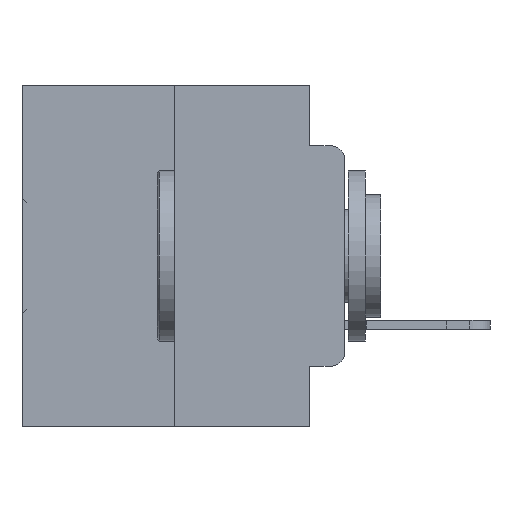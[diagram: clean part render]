
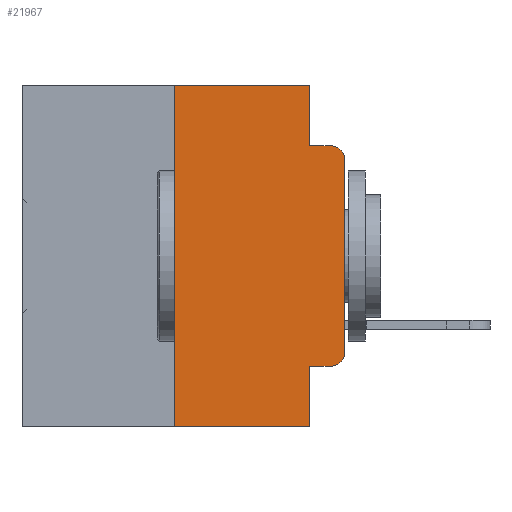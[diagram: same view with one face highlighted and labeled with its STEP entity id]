
A CAD part, left-side view. The second image highlights one B-rep face of the part: STEP entity #21967.
In plain terms, the highlighted planar face has unit normal (-1, 0, 0).
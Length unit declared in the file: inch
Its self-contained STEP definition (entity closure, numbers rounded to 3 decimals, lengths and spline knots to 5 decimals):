
#9 = VECTOR ( 'NONE', #4229, 39.37008 ) ;
#162 = CARTESIAN_POINT ( 'NONE',  ( 0., 0.02, -0.0885 ) ) ;
#544 = CARTESIAN_POINT ( 'NONE',  ( 0., 0.473, -0.5 ) ) ;
#955 = LINE ( 'NONE', #9990, #9 ) ;
#1294 = ORIENTED_EDGE ( 'NONE', *, *, #5233, .T. ) ;
#1301 = EDGE_CURVE ( 'NONE', #25067, #18121, #32354, .T. ) ;
#3292 = ORIENTED_EDGE ( 'NONE', *, *, #1301, .T. ) ;
#3475 = VERTEX_POINT ( 'NONE', #28756 ) ;
#3494 = DIRECTION ( 'NONE',  ( 0., -1., 0. ) ) ;
#4229 = DIRECTION ( 'NONE',  ( 0., -1., 0. ) ) ;
#4301 = VERTEX_POINT ( 'NONE', #18008 ) ;
#4557 = LINE ( 'NONE', #26283, #11226 ) ;
#4990 = ORIENTED_EDGE ( 'NONE', *, *, #32111, .F. ) ;
#5233 = EDGE_CURVE ( 'NONE', #30755, #25067, #18226, .T. ) ;
#5246 = ORIENTED_EDGE ( 'NONE', *, *, #25232, .F. ) ;
#5664 = VERTEX_POINT ( 'NONE', #18319 ) ;
#7250 = CARTESIAN_POINT ( 'NONE',  ( 0., 0.473, 0. ) ) ;
#8389 = EDGE_CURVE ( 'NONE', #4301, #11803, #9039, .T. ) ;
#8598 = LINE ( 'NONE', #19169, #34910 ) ;
#9039 = CIRCLE ( 'NONE', #10577, 0.02 ) ;
#9617 = CARTESIAN_POINT ( 'NONE',  ( 0., 0.02, -0.4115 ) ) ;
#9990 = CARTESIAN_POINT ( 'NONE',  ( 0., 0.473, 0. ) ) ;
#10044 = DIRECTION ( 'NONE',  ( 0., 0., 1. ) ) ;
#10074 = DIRECTION ( 'NONE',  ( 1., 0., 0. ) ) ;
#10155 = VECTOR ( 'NONE', #30613, 39.37008 ) ;
#10577 = AXIS2_PLACEMENT_3D ( 'NONE', #11622, #11499, #11469 ) ;
#10914 = EDGE_CURVE ( 'NONE', #30755, #3475, #26461, .T. ) ;
#11226 = VECTOR ( 'NONE', #28831, 39.37008 ) ;
#11469 = DIRECTION ( 'NONE',  ( 0., 0., -1. ) ) ;
#11499 = DIRECTION ( 'NONE',  ( -1., 0., 0. ) ) ;
#11622 = CARTESIAN_POINT ( 'NONE',  ( 0., 0.02, -0.1085 ) ) ;
#11803 = VERTEX_POINT ( 'NONE', #162 ) ;
#12733 = EDGE_CURVE ( 'NONE', #5664, #14747, #30363, .T. ) ;
#13127 = VECTOR ( 'NONE', #3494, 39.37008 ) ;
#13420 = DIRECTION ( 'NONE',  ( 0., 0., -1. ) ) ;
#13431 = CARTESIAN_POINT ( 'NONE',  ( 0., 0.051, 0. ) ) ;
#13567 = ORIENTED_EDGE ( 'NONE', *, *, #26563, .F. ) ;
#13974 = CARTESIAN_POINT ( 'NONE',  ( 0., 0., -0.3915 ) ) ;
#14747 = VERTEX_POINT ( 'NONE', #23717 ) ;
#15728 = EDGE_CURVE ( 'NONE', #18121, #4301, #8598, .T. ) ;
#16088 = CARTESIAN_POINT ( 'NONE',  ( 0., 0.051, 0. ) ) ;
#18008 = CARTESIAN_POINT ( 'NONE',  ( 0., 0., -0.1085 ) ) ;
#18121 = VERTEX_POINT ( 'NONE', #13974 ) ;
#18226 = LINE ( 'NONE', #30571, #10155 ) ;
#18319 = CARTESIAN_POINT ( 'NONE',  ( 0., 0.25, -0.5 ) ) ;
#19169 = CARTESIAN_POINT ( 'NONE',  ( 0., 0., 0. ) ) ;
#19987 = VERTEX_POINT ( 'NONE', #16088 ) ;
#20302 = VECTOR ( 'NONE', #13420, 39.37008 ) ;
#20640 = CARTESIAN_POINT ( 'NONE',  ( 0., 0.02, -0.3915 ) ) ;
#21967 = ADVANCED_FACE ( 'NONE', ( #34445 ), #23293, .F. ) ;
#22881 = ORIENTED_EDGE ( 'NONE', *, *, #15728, .T. ) ;
#23192 = EDGE_LOOP ( 'NONE', ( #22881, #25909, #4990, #5246, #13567, #23478, #29846, #33278, #1294, #3292 ) ) ;
#23293 = PLANE ( 'NONE',  #31163 ) ;
#23458 = VECTOR ( 'NONE', #10044, 39.37008 ) ;
#23478 = ORIENTED_EDGE ( 'NONE', *, *, #12733, .F. ) ;
#23717 = CARTESIAN_POINT ( 'NONE',  ( 0., 0.25, 0. ) ) ;
#25067 = VERTEX_POINT ( 'NONE', #9617 ) ;
#25126 = CARTESIAN_POINT ( 'NONE',  ( 0., 0.051, -0.0885 ) ) ;
#25232 = EDGE_CURVE ( 'NONE', #19987, #31895, #4557, .T. ) ;
#25909 = ORIENTED_EDGE ( 'NONE', *, *, #8389, .T. ) ;
#25988 = CARTESIAN_POINT ( 'NONE',  ( 0., 0.051, -0.4115 ) ) ;
#26283 = CARTESIAN_POINT ( 'NONE',  ( 0., 0.051, 0. ) ) ;
#26461 = LINE ( 'NONE', #13431, #20302 ) ;
#26563 = EDGE_CURVE ( 'NONE', #14747, #19987, #955, .T. ) ;
#27299 = LINE ( 'NONE', #31051, #33265 ) ;
#28134 = DIRECTION ( 'NONE',  ( 0., 0., -1. ) ) ;
#28168 = DIRECTION ( 'NONE',  ( -1., 0., 0. ) ) ;
#28610 = DIRECTION ( 'NONE',  ( 0., 0., -1. ) ) ;
#28756 = CARTESIAN_POINT ( 'NONE',  ( 0., 0.051, -0.5 ) ) ;
#28776 = LINE ( 'NONE', #544, #13127 ) ;
#28831 = DIRECTION ( 'NONE',  ( 0., 0., -1. ) ) ;
#29846 = ORIENTED_EDGE ( 'NONE', *, *, #30192, .T. ) ;
#29899 = AXIS2_PLACEMENT_3D ( 'NONE', #20640, #28168, #28134 ) ;
#30192 = EDGE_CURVE ( 'NONE', #5664, #3475, #28776, .T. ) ;
#30363 = LINE ( 'NONE', #33610, #23458 ) ;
#30571 = CARTESIAN_POINT ( 'NONE',  ( 0., 0.051, -0.4115 ) ) ;
#30613 = DIRECTION ( 'NONE',  ( 0., -1., 0. ) ) ;
#30755 = VERTEX_POINT ( 'NONE', #25988 ) ;
#31051 = CARTESIAN_POINT ( 'NONE',  ( 0., 0.051, -0.0885 ) ) ;
#31163 = AXIS2_PLACEMENT_3D ( 'NONE', #7250, #10074, #28610 ) ;
#31895 = VERTEX_POINT ( 'NONE', #25126 ) ;
#32111 = EDGE_CURVE ( 'NONE', #31895, #11803, #27299, .T. ) ;
#32354 = CIRCLE ( 'NONE', #29899, 0.02 ) ;
#33265 = VECTOR ( 'NONE', #33596, 39.37008 ) ;
#33278 = ORIENTED_EDGE ( 'NONE', *, *, #10914, .F. ) ;
#33596 = DIRECTION ( 'NONE',  ( 0., -1., 0. ) ) ;
#33610 = CARTESIAN_POINT ( 'NONE',  ( 0., 0.25, 0. ) ) ;
#34445 = FACE_OUTER_BOUND ( 'NONE', #23192, .T. ) ;
#34592 = DIRECTION ( 'NONE',  ( 0., 0., 1. ) ) ;
#34910 = VECTOR ( 'NONE', #34592, 39.37008 ) ;
